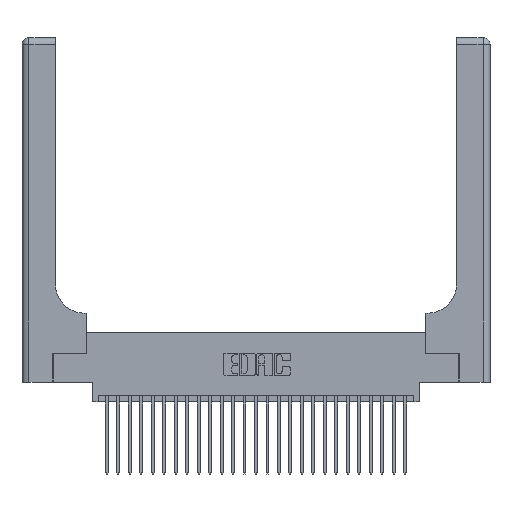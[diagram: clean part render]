
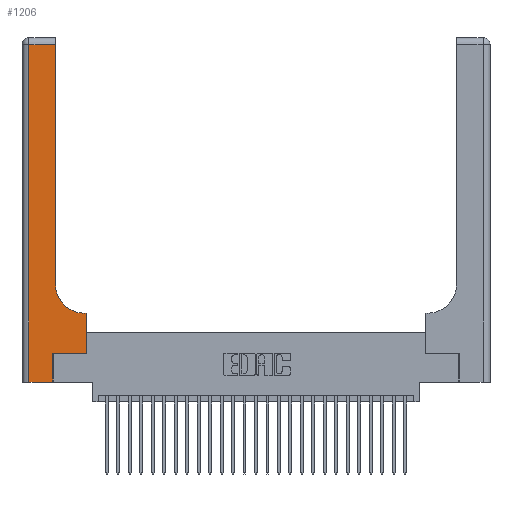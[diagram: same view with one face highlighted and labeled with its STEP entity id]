
A CAD part, top view. The second image highlights one B-rep face of the part: STEP entity #1206.
In plain terms, the highlighted planar face has unit normal (0, 0, 1).
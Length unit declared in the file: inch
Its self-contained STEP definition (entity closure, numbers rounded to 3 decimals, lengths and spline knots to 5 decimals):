
#486 = ORIENTED_EDGE ( 'NONE', *, *, #18346, .T. ) ;
#574 = CARTESIAN_POINT ( 'NONE',  ( 0.5585, 0.25, 0.37 ) ) ;
#651 = ORIENTED_EDGE ( 'NONE', *, *, #18984, .T. ) ;
#744 = VERTEX_POINT ( 'NONE', #4444 ) ;
#1206 = ADVANCED_FACE ( 'NONE', ( #4650 ), #6422, .F. ) ;
#2054 = CIRCLE ( 'NONE', #24845, 0.25 ) ;
#2699 = VECTOR ( 'NONE', #22275, 39.37008 ) ;
#3639 = AXIS2_PLACEMENT_3D ( 'NONE', #8667, #16126, #18478 ) ;
#4381 = VECTOR ( 'NONE', #10027, 39.37008 ) ;
#4444 = CARTESIAN_POINT ( 'NONE',  ( 0.269, 0., 0.37 ) ) ;
#4632 = DIRECTION ( 'NONE',  ( 1., 0., 0. ) ) ;
#4650 = FACE_OUTER_BOUND ( 'NONE', #6885, .T. ) ;
#5292 = ORIENTED_EDGE ( 'NONE', *, *, #14128, .T. ) ;
#5444 = EDGE_CURVE ( 'NONE', #15755, #5803, #6376, .T. ) ;
#5792 = ORIENTED_EDGE ( 'NONE', *, *, #9317, .T. ) ;
#5803 = VERTEX_POINT ( 'NONE', #8759 ) ;
#6109 = EDGE_CURVE ( 'NONE', #6563, #23817, #14945, .T. ) ;
#6158 = LINE ( 'NONE', #13777, #2699 ) ;
#6376 = LINE ( 'NONE', #574, #23617 ) ;
#6422 = PLANE ( 'NONE',  #3639 ) ;
#6563 = VERTEX_POINT ( 'NONE', #26272 ) ;
#6608 = EDGE_CURVE ( 'NONE', #7406, #744, #11849, .T. ) ;
#6885 = EDGE_LOOP ( 'NONE', ( #486, #18933, #651, #19799, #10820, #5292, #25901, #16351, #5792 ) ) ;
#7167 = DIRECTION ( 'NONE',  ( 0., 0., -1. ) ) ;
#7406 = VERTEX_POINT ( 'NONE', #7626 ) ;
#7626 = CARTESIAN_POINT ( 'NONE',  ( 0.06, 0., 0.37 ) ) ;
#8335 = EDGE_CURVE ( 'NONE', #744, #12851, #20742, .T. ) ;
#8667 = CARTESIAN_POINT ( 'NONE',  ( 0., 3., 0.37 ) ) ;
#8759 = CARTESIAN_POINT ( 'NONE',  ( 0.5585, 0.6, 0.37 ) ) ;
#8795 = VECTOR ( 'NONE', #21558, 39.37008 ) ;
#9317 = EDGE_CURVE ( 'NONE', #19746, #17377, #2054, .T. ) ;
#9821 = VECTOR ( 'NONE', #25038, 39.37008 ) ;
#9842 = LINE ( 'NONE', #28015, #8795 ) ;
#10027 = DIRECTION ( 'NONE',  ( 0., -1., 0. ) ) ;
#10268 = CARTESIAN_POINT ( 'NONE',  ( 0.5585, 0.25, 0.37 ) ) ;
#10820 = ORIENTED_EDGE ( 'NONE', *, *, #8335, .T. ) ;
#11849 = LINE ( 'NONE', #27026, #18711 ) ;
#12851 = VERTEX_POINT ( 'NONE', #13253 ) ;
#13253 = CARTESIAN_POINT ( 'NONE',  ( 0.269, 0.25, 0.37 ) ) ;
#13777 = CARTESIAN_POINT ( 'NONE',  ( 0.2915, 3., 0.37 ) ) ;
#14128 = EDGE_CURVE ( 'NONE', #12851, #15755, #22767, .T. ) ;
#14804 = VECTOR ( 'NONE', #25144, 39.37008 ) ;
#14945 = LINE ( 'NONE', #27336, #9821 ) ;
#15192 = VECTOR ( 'NONE', #22065, 39.37008 ) ;
#15401 = LINE ( 'NONE', #23190, #4381 ) ;
#15755 = VERTEX_POINT ( 'NONE', #10268 ) ;
#16115 = DIRECTION ( 'NONE',  ( 1., 0., 0. ) ) ;
#16126 = DIRECTION ( 'NONE',  ( 0., 0., -1. ) ) ;
#16351 = ORIENTED_EDGE ( 'NONE', *, *, #26974, .T. ) ;
#17377 = VERTEX_POINT ( 'NONE', #19416 ) ;
#18346 = EDGE_CURVE ( 'NONE', #17377, #6563, #6158, .T. ) ;
#18425 = CARTESIAN_POINT ( 'NONE',  ( 0.06, 2.94, 0.37 ) ) ;
#18478 = DIRECTION ( 'NONE',  ( -1., 0., 0. ) ) ;
#18711 = VECTOR ( 'NONE', #4632, 39.37008 ) ;
#18933 = ORIENTED_EDGE ( 'NONE', *, *, #6109, .T. ) ;
#18984 = EDGE_CURVE ( 'NONE', #23817, #7406, #15401, .T. ) ;
#19416 = CARTESIAN_POINT ( 'NONE',  ( 0.2915, 0.85, 0.37 ) ) ;
#19746 = VERTEX_POINT ( 'NONE', #27413 ) ;
#19799 = ORIENTED_EDGE ( 'NONE', *, *, #6608, .T. ) ;
#19936 = CARTESIAN_POINT ( 'NONE',  ( 0.269, 0., 0.37 ) ) ;
#20664 = CARTESIAN_POINT ( 'NONE',  ( 0.5415, 0.85, 0.37 ) ) ;
#20742 = LINE ( 'NONE', #19936, #15192 ) ;
#20777 = CARTESIAN_POINT ( 'NONE',  ( 0.269, 0.25, 0.37 ) ) ;
#21558 = DIRECTION ( 'NONE',  ( -1., 0., 0. ) ) ;
#22065 = DIRECTION ( 'NONE',  ( 0., 1., 0. ) ) ;
#22275 = DIRECTION ( 'NONE',  ( 0., 1., 0. ) ) ;
#22657 = DIRECTION ( 'NONE',  ( 0., 1., 0. ) ) ;
#22767 = LINE ( 'NONE', #20777, #14804 ) ;
#23190 = CARTESIAN_POINT ( 'NONE',  ( 0.06, 3., 0.37 ) ) ;
#23617 = VECTOR ( 'NONE', #22657, 39.37008 ) ;
#23817 = VERTEX_POINT ( 'NONE', #18425 ) ;
#24845 = AXIS2_PLACEMENT_3D ( 'NONE', #20664, #7167, #16115 ) ;
#25038 = DIRECTION ( 'NONE',  ( -1., 0., 0. ) ) ;
#25144 = DIRECTION ( 'NONE',  ( 1., 0., 0. ) ) ;
#25901 = ORIENTED_EDGE ( 'NONE', *, *, #5444, .T. ) ;
#26272 = CARTESIAN_POINT ( 'NONE',  ( 0.2915, 2.94, 0.37 ) ) ;
#26974 = EDGE_CURVE ( 'NONE', #5803, #19746, #9842, .T. ) ;
#27026 = CARTESIAN_POINT ( 'NONE',  ( 0., 0., 0.37 ) ) ;
#27336 = CARTESIAN_POINT ( 'NONE',  ( 0., 2.94, 0.37 ) ) ;
#27413 = CARTESIAN_POINT ( 'NONE',  ( 0.5415, 0.6, 0.37 ) ) ;
#28015 = CARTESIAN_POINT ( 'NONE',  ( 0.2915, 0.6, 0.37 ) ) ;
